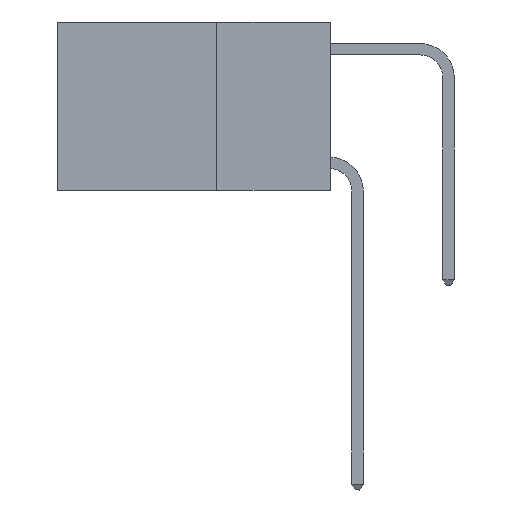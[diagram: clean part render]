
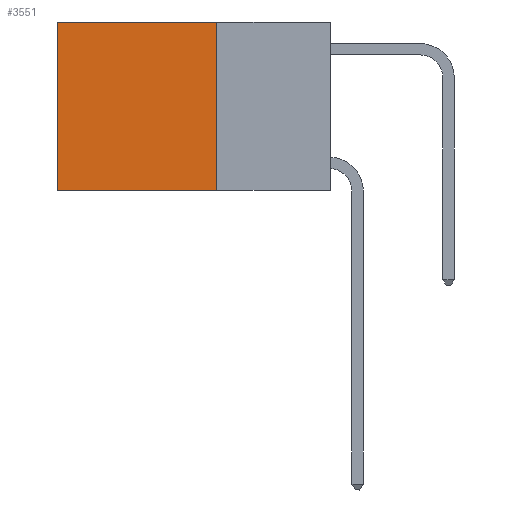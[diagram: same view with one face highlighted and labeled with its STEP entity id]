
A CAD part, left-side view. The second image highlights one B-rep face of the part: STEP entity #3551.
In plain terms, the highlighted planar face has unit normal (-1, 0, 0).
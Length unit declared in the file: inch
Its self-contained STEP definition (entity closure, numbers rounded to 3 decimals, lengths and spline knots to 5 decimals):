
#600 = CARTESIAN_POINT ( 'NONE',  ( 0.2625, 0.25, 0. ) ) ;
#979 = CARTESIAN_POINT ( 'NONE',  ( 0.2625, 0.25, -0.37 ) ) ;
#1364 = VERTEX_POINT ( 'NONE', #600 ) ;
#1512 = CARTESIAN_POINT ( 'NONE',  ( 0.2625, 0.25, 0. ) ) ;
#1945 = ORIENTED_EDGE ( 'NONE', *, *, #17758, .F. ) ;
#2933 = DIRECTION ( 'NONE',  ( 0., 0., -1. ) ) ;
#3298 = CARTESIAN_POINT ( 'NONE',  ( 0.2625, 0.6, -0.37 ) ) ;
#3518 = CARTESIAN_POINT ( 'NONE',  ( 0.2625, 0.25, 0. ) ) ;
#3551 = ADVANCED_FACE ( 'NONE', ( #14424 ), #11167, .F. ) ;
#3596 = EDGE_CURVE ( 'NONE', #8758, #18714, #18245, .T. ) ;
#3827 = LINE ( 'NONE', #10920, #11448 ) ;
#4159 = LINE ( 'NONE', #3518, #16640 ) ;
#5174 = DIRECTION ( 'NONE',  ( 0., 1., 0. ) ) ;
#7724 = EDGE_CURVE ( 'NONE', #20249, #18714, #3827, .T. ) ;
#8295 = CARTESIAN_POINT ( 'NONE',  ( 0.2625, 0.25, 0. ) ) ;
#8758 = VERTEX_POINT ( 'NONE', #13949 ) ;
#10595 = ORIENTED_EDGE ( 'NONE', *, *, #7724, .F. ) ;
#10920 = CARTESIAN_POINT ( 'NONE',  ( 0.2625, 0.25, -0.37 ) ) ;
#11167 = PLANE ( 'NONE',  #20380 ) ;
#11236 = DIRECTION ( 'NONE',  ( 1., 0., 0. ) ) ;
#11448 = VECTOR ( 'NONE', #12543, 39.37008 ) ;
#11727 = EDGE_LOOP ( 'NONE', ( #15148, #10595, #1945, #19786 ) ) ;
#12543 = DIRECTION ( 'NONE',  ( 0., 1., 0. ) ) ;
#13284 = DIRECTION ( 'NONE',  ( 0., 0., -1. ) ) ;
#13949 = CARTESIAN_POINT ( 'NONE',  ( 0.2625, 0.6, 0. ) ) ;
#14424 = FACE_OUTER_BOUND ( 'NONE', #11727, .T. ) ;
#15148 = ORIENTED_EDGE ( 'NONE', *, *, #3596, .T. ) ;
#16142 = DIRECTION ( 'NONE',  ( 0., 0., -1. ) ) ;
#16148 = VECTOR ( 'NONE', #5174, 39.37008 ) ;
#16640 = VECTOR ( 'NONE', #13284, 39.37008 ) ;
#17179 = EDGE_CURVE ( 'NONE', #1364, #8758, #21010, .T. ) ;
#17758 = EDGE_CURVE ( 'NONE', #1364, #20249, #4159, .T. ) ;
#18245 = LINE ( 'NONE', #21073, #19271 ) ;
#18714 = VERTEX_POINT ( 'NONE', #3298 ) ;
#19271 = VECTOR ( 'NONE', #16142, 39.37008 ) ;
#19786 = ORIENTED_EDGE ( 'NONE', *, *, #17179, .T. ) ;
#20249 = VERTEX_POINT ( 'NONE', #979 ) ;
#20380 = AXIS2_PLACEMENT_3D ( 'NONE', #1512, #11236, #2933 ) ;
#21010 = LINE ( 'NONE', #8295, #16148 ) ;
#21073 = CARTESIAN_POINT ( 'NONE',  ( 0.2625, 0.6, 0. ) ) ;
